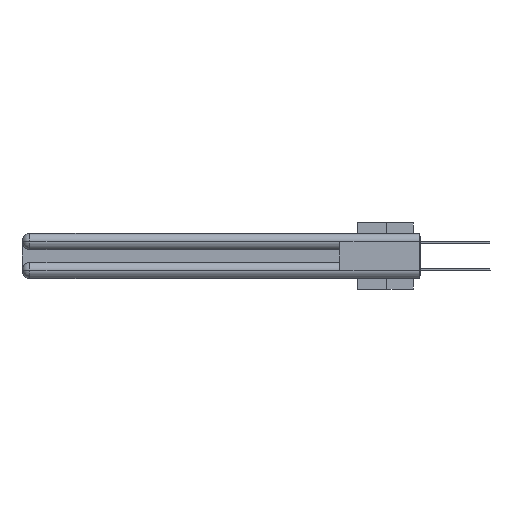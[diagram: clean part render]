
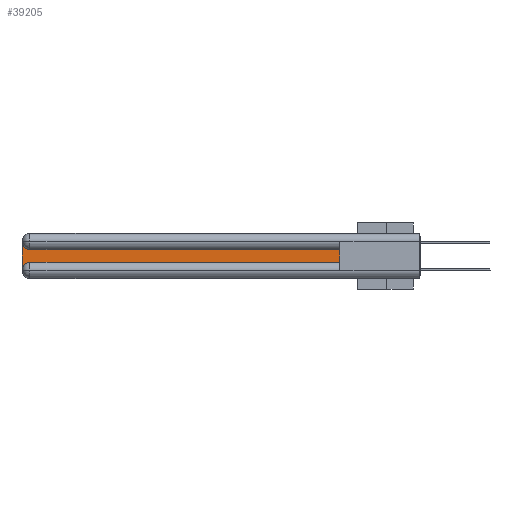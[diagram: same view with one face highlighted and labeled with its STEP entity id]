
A CAD part, left-side view. The second image highlights one B-rep face of the part: STEP entity #39205.
In plain terms, the highlighted planar face has unit normal (-1, 0, 0).
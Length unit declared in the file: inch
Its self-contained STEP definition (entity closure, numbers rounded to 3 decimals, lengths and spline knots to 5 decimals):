
#137 = CARTESIAN_POINT ( 'NONE',  ( 0.075, 3., -0.0625 ) ) ;
#1035 = VERTEX_POINT ( 'NONE', #2833 ) ;
#1263 = CARTESIAN_POINT ( 'NONE',  ( 0.075, 0.6, -0.1225 ) ) ;
#1761 = CARTESIAN_POINT ( 'NONE',  ( 0.075, 3., -0.2775 ) ) ;
#2094 = DIRECTION ( 'NONE',  ( 0., -1., 0. ) ) ;
#2281 = CARTESIAN_POINT ( 'NONE',  ( 0.075, 3., -0.1225 ) ) ;
#2833 = CARTESIAN_POINT ( 'NONE',  ( 0.075, 2.94, -0.2175 ) ) ;
#3072 = EDGE_CURVE ( 'NONE', #1035, #14865, #24295, .T. ) ;
#3204 = VECTOR ( 'NONE', #10720, 39.37008 ) ;
#3747 = ORIENTED_EDGE ( 'NONE', *, *, #3072, .T. ) ;
#4918 = EDGE_CURVE ( 'NONE', #30589, #34496, #20672, .T. ) ;
#6390 = CARTESIAN_POINT ( 'NONE',  ( 0.075, 2.94, -0.2775 ) ) ;
#6988 = DIRECTION ( 'NONE',  ( 1., 0., 0. ) ) ;
#8326 = VERTEX_POINT ( 'NONE', #1761 ) ;
#8364 = DIRECTION ( 'NONE',  ( 1., 0., 0. ) ) ;
#10720 = DIRECTION ( 'NONE',  ( 0., 0., -1. ) ) ;
#10807 = CARTESIAN_POINT ( 'NONE',  ( 0.075, 0.6, -0.2175 ) ) ;
#10998 = PLANE ( 'NONE',  #30255 ) ;
#11762 = EDGE_CURVE ( 'NONE', #37201, #8326, #23260, .T. ) ;
#11922 = DIRECTION ( 'NONE',  ( 1., 0., 0. ) ) ;
#12033 = AXIS2_PLACEMENT_3D ( 'NONE', #33975, #11922, #36816 ) ;
#12835 = CARTESIAN_POINT ( 'NONE',  ( 0.075, 2.94, -0.1225 ) ) ;
#13355 = CARTESIAN_POINT ( 'NONE',  ( 0.075, 3., -0.2175 ) ) ;
#13792 = DIRECTION ( 'NONE',  ( 0., 1., 0. ) ) ;
#14865 = VERTEX_POINT ( 'NONE', #31988 ) ;
#16990 = CARTESIAN_POINT ( 'NONE',  ( 0.075, 0.6, -0.1225 ) ) ;
#18722 = DIRECTION ( 'NONE',  ( 0., 0., -1. ) ) ;
#18749 = ORIENTED_EDGE ( 'NONE', *, *, #11762, .T. ) ;
#19356 = VECTOR ( 'NONE', #2094, 39.37008 ) ;
#20056 = EDGE_CURVE ( 'NONE', #8326, #1035, #23725, .T. ) ;
#20672 = LINE ( 'NONE', #1263, #31747 ) ;
#21932 = DIRECTION ( 'NONE',  ( 0., 0., 1. ) ) ;
#23260 = LINE ( 'NONE', #13355, #3204 ) ;
#23725 = CIRCLE ( 'NONE', #26322, 0.06 ) ;
#24179 = VECTOR ( 'NONE', #21932, 39.37008 ) ;
#24295 = LINE ( 'NONE', #10807, #19356 ) ;
#26163 = FACE_OUTER_BOUND ( 'NONE', #29348, .T. ) ;
#26322 = AXIS2_PLACEMENT_3D ( 'NONE', #6390, #6988, #18722 ) ;
#26363 = DIRECTION ( 'NONE',  ( 0., 0., -1. ) ) ;
#27641 = ORIENTED_EDGE ( 'NONE', *, *, #4918, .T. ) ;
#28183 = CIRCLE ( 'NONE', #12033, 0.06 ) ;
#28630 = EDGE_CURVE ( 'NONE', #14865, #30589, #32019, .T. ) ;
#28990 = CARTESIAN_POINT ( 'NONE',  ( 0.075, 0.6, -0.2175 ) ) ;
#29348 = EDGE_LOOP ( 'NONE', ( #27641, #37449, #18749, #30087, #3747, #30395 ) ) ;
#30087 = ORIENTED_EDGE ( 'NONE', *, *, #20056, .T. ) ;
#30255 = AXIS2_PLACEMENT_3D ( 'NONE', #2281, #8364, #26363 ) ;
#30395 = ORIENTED_EDGE ( 'NONE', *, *, #28630, .T. ) ;
#30589 = VERTEX_POINT ( 'NONE', #16990 ) ;
#31747 = VECTOR ( 'NONE', #13792, 39.37008 ) ;
#31988 = CARTESIAN_POINT ( 'NONE',  ( 0.075, 0.6, -0.2175 ) ) ;
#32019 = LINE ( 'NONE', #28990, #24179 ) ;
#33975 = CARTESIAN_POINT ( 'NONE',  ( 0.075, 2.94, -0.0625 ) ) ;
#34496 = VERTEX_POINT ( 'NONE', #12835 ) ;
#36794 = EDGE_CURVE ( 'NONE', #34496, #37201, #28183, .T. ) ;
#36816 = DIRECTION ( 'NONE',  ( 0., 0., -1. ) ) ;
#37201 = VERTEX_POINT ( 'NONE', #137 ) ;
#37449 = ORIENTED_EDGE ( 'NONE', *, *, #36794, .T. ) ;
#39205 = ADVANCED_FACE ( 'NONE', ( #26163 ), #10998, .F. ) ;
